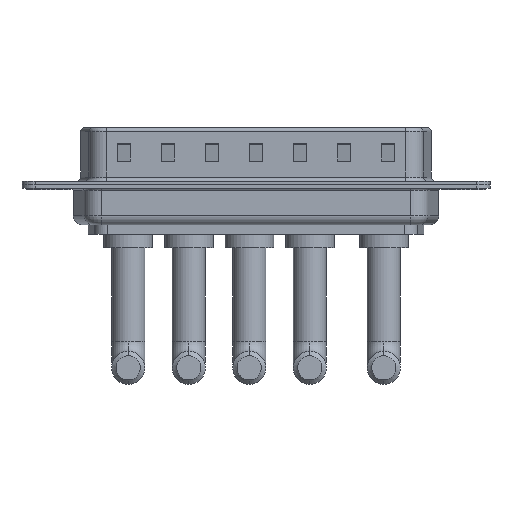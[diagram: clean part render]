
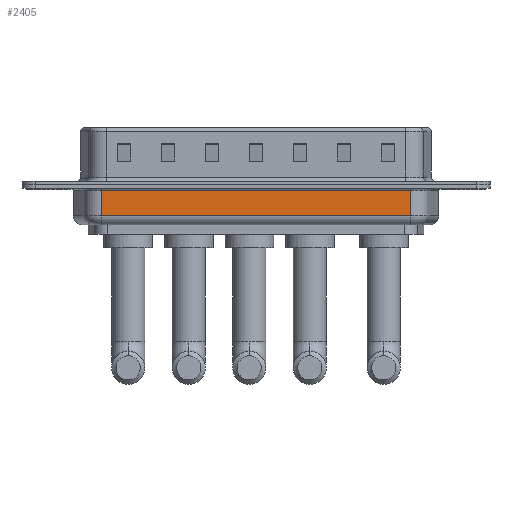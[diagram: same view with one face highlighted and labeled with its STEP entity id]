
A CAD part, front view. The second image highlights one B-rep face of the part: STEP entity #2405.
In plain terms, the highlighted planar face has unit normal (0, -1, 0).
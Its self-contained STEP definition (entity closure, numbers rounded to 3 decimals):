
#718 = CARTESIAN_POINT ( 'NONE',  ( 41.044, -5.35, -4.5 ) ) ;
#776 = ORIENTED_EDGE ( 'NONE', *, *, #5511, .T. ) ;
#1240 = LINE ( 'NONE', #2207, #7228 ) ;
#2207 = CARTESIAN_POINT ( 'NONE',  ( 6.006, -5.35, -4.5 ) ) ;
#2405 = ADVANCED_FACE ( 'NONE', ( #12391 ), #12586, .F. ) ;
#2443 = DIRECTION ( 'NONE',  ( -1., 0., 0. ) ) ;
#3253 = AXIS2_PLACEMENT_3D ( 'NONE', #3879, #7561, #12454 ) ;
#3657 = VERTEX_POINT ( 'NONE', #8514 ) ;
#3879 = CARTESIAN_POINT ( 'NONE',  ( 6.006, -5.35, -4.5 ) ) ;
#4034 = VECTOR ( 'NONE', #11768, 1000. ) ;
#4136 = DIRECTION ( 'NONE',  ( 0., 0., 1. ) ) ;
#4144 = VECTOR ( 'NONE', #2443, 1000. ) ;
#4243 = CARTESIAN_POINT ( 'NONE',  ( 41.044, -5.35, -0.65 ) ) ;
#4977 = LINE ( 'NONE', #10816, #4034 ) ;
#5511 = EDGE_CURVE ( 'NONE', #10281, #7118, #5517, .T. ) ;
#5517 = LINE ( 'NONE', #10099, #4144 ) ;
#5952 = EDGE_LOOP ( 'NONE', ( #6953, #12484, #9324, #776 ) ) ;
#6709 = VERTEX_POINT ( 'NONE', #7905 ) ;
#6953 = ORIENTED_EDGE ( 'NONE', *, *, #8368, .F. ) ;
#7118 = VERTEX_POINT ( 'NONE', #8833 ) ;
#7228 = VECTOR ( 'NONE', #4136, 1000. ) ;
#7561 = DIRECTION ( 'NONE',  ( 0., 1., 0. ) ) ;
#7905 = CARTESIAN_POINT ( 'NONE',  ( 41.044, -5.35, -3.5 ) ) ;
#8368 = EDGE_CURVE ( 'NONE', #3657, #7118, #1240, .T. ) ;
#8514 = CARTESIAN_POINT ( 'NONE',  ( 6.006, -5.35, -3.5 ) ) ;
#8833 = CARTESIAN_POINT ( 'NONE',  ( 6.006, -5.35, -0.65 ) ) ;
#9297 = VECTOR ( 'NONE', #11491, 1000. ) ;
#9324 = ORIENTED_EDGE ( 'NONE', *, *, #10056, .T. ) ;
#9375 = LINE ( 'NONE', #718, #9297 ) ;
#9787 = EDGE_CURVE ( 'NONE', #3657, #6709, #4977, .T. ) ;
#10056 = EDGE_CURVE ( 'NONE', #6709, #10281, #9375, .T. ) ;
#10099 = CARTESIAN_POINT ( 'NONE',  ( 6.006, -5.35, -0.65 ) ) ;
#10281 = VERTEX_POINT ( 'NONE', #4243 ) ;
#10816 = CARTESIAN_POINT ( 'NONE',  ( 6.006, -5.35, -3.5 ) ) ;
#11491 = DIRECTION ( 'NONE',  ( 0., 0., 1. ) ) ;
#11768 = DIRECTION ( 'NONE',  ( 1., 0., 0. ) ) ;
#12391 = FACE_OUTER_BOUND ( 'NONE', #5952, .T. ) ;
#12454 = DIRECTION ( 'NONE',  ( 0., 0., 1. ) ) ;
#12484 = ORIENTED_EDGE ( 'NONE', *, *, #9787, .T. ) ;
#12586 = PLANE ( 'NONE',  #3253 ) ;
